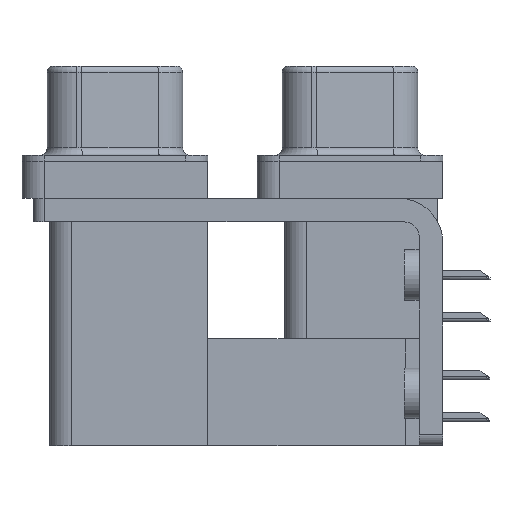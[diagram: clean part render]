
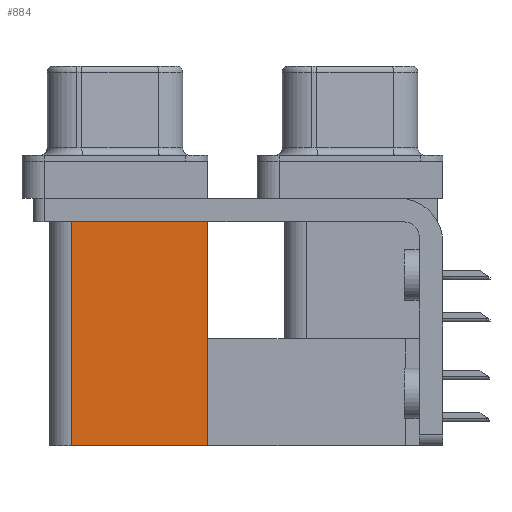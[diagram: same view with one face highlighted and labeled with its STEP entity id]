
A CAD part, left-side view. The second image highlights one B-rep face of the part: STEP entity #884.
In plain terms, the highlighted planar face has unit normal (-1, 0, 0).
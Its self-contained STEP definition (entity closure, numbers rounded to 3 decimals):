
#385 = VERTEX_POINT ( 'NONE', #28487 ) ;
#884 = ADVANCED_FACE ( 'NONE', ( #28300 ), #18936, .F. ) ;
#1117 = LINE ( 'NONE', #1300, #21589 ) ;
#1300 = CARTESIAN_POINT ( 'NONE',  ( 3.765, 9.6, -19.2 ) ) ;
#3587 = DIRECTION ( 'NONE',  ( 0., 0., 1. ) ) ;
#4211 = DIRECTION ( 'NONE',  ( 0., 0., 1. ) ) ;
#4273 = CARTESIAN_POINT ( 'NONE',  ( 3.765, 18.8, -19.2 ) ) ;
#5288 = VECTOR ( 'NONE', #3587, 1000. ) ;
#6530 = CARTESIAN_POINT ( 'NONE',  ( 3.765, 9.6, -19.2 ) ) ;
#7062 = LINE ( 'NONE', #11535, #15848 ) ;
#8043 = EDGE_CURVE ( 'NONE', #18633, #22393, #30780, .T. ) ;
#8106 = DIRECTION ( 'NONE',  ( 0., 1., 0. ) ) ;
#10797 = EDGE_LOOP ( 'NONE', ( #18299, #20343, #23819, #11727 ) ) ;
#11535 = CARTESIAN_POINT ( 'NONE',  ( 3.765, 18.8, -19.2 ) ) ;
#11727 = ORIENTED_EDGE ( 'NONE', *, *, #8043, .T. ) ;
#11937 = DIRECTION ( 'NONE',  ( 1., 0., 0. ) ) ;
#15413 = LINE ( 'NONE', #27195, #29572 ) ;
#15848 = VECTOR ( 'NONE', #4211, 1000. ) ;
#18299 = ORIENTED_EDGE ( 'NONE', *, *, #24344, .T. ) ;
#18633 = VERTEX_POINT ( 'NONE', #20008 ) ;
#18779 = DIRECTION ( 'NONE',  ( 0., 0., -1. ) ) ;
#18936 = PLANE ( 'NONE',  #31181 ) ;
#20008 = CARTESIAN_POINT ( 'NONE',  ( 3.765, 9.6, -19.2 ) ) ;
#20326 = DIRECTION ( 'NONE',  ( 0., 1., 0. ) ) ;
#20343 = ORIENTED_EDGE ( 'NONE', *, *, #26075, .F. ) ;
#20728 = CARTESIAN_POINT ( 'NONE',  ( 3.765, 9.6, -2.5 ) ) ;
#21589 = VECTOR ( 'NONE', #8106, 1000. ) ;
#22393 = VERTEX_POINT ( 'NONE', #20728 ) ;
#23265 = VERTEX_POINT ( 'NONE', #4273 ) ;
#23819 = ORIENTED_EDGE ( 'NONE', *, *, #28213, .F. ) ;
#24344 = EDGE_CURVE ( 'NONE', #22393, #385, #15413, .T. ) ;
#26075 = EDGE_CURVE ( 'NONE', #23265, #385, #7062, .T. ) ;
#27195 = CARTESIAN_POINT ( 'NONE',  ( 3.765, 9.6, -2.5 ) ) ;
#28213 = EDGE_CURVE ( 'NONE', #18633, #23265, #1117, .T. ) ;
#28300 = FACE_OUTER_BOUND ( 'NONE', #10797, .T. ) ;
#28487 = CARTESIAN_POINT ( 'NONE',  ( 3.765, 18.8, -2.5 ) ) ;
#29572 = VECTOR ( 'NONE', #20326, 1000. ) ;
#30299 = CARTESIAN_POINT ( 'NONE',  ( 3.765, 9.6, -19.2 ) ) ;
#30780 = LINE ( 'NONE', #30299, #5288 ) ;
#31181 = AXIS2_PLACEMENT_3D ( 'NONE', #6530, #11937, #18779 ) ;
